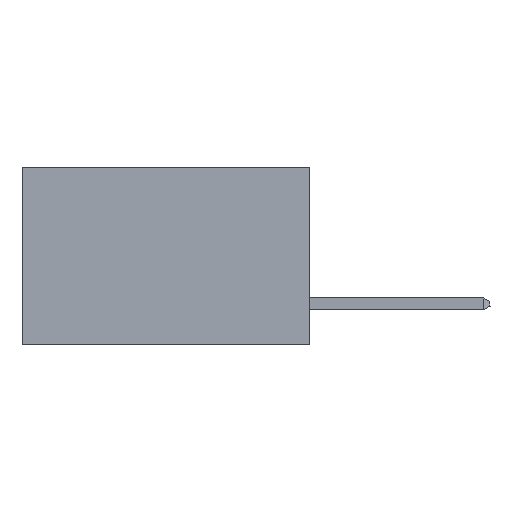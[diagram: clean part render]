
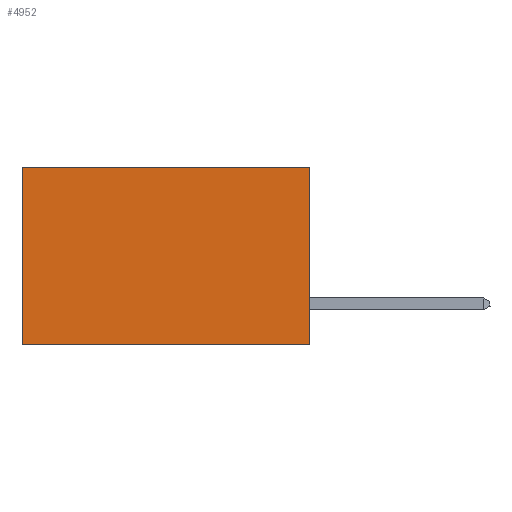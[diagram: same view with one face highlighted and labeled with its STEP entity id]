
A CAD part, left-side view. The second image highlights one B-rep face of the part: STEP entity #4952.
In plain terms, the highlighted planar face has unit normal (-1, 0, 0).
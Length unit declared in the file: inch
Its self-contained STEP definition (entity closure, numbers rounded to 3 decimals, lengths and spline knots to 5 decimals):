
#115 = DIRECTION ( 'NONE',  ( 0., 1., 0. ) ) ;
#611 = ORIENTED_EDGE ( 'NONE', *, *, #8320, .T. ) ;
#1024 = EDGE_CURVE ( 'NONE', #9389, #12700, #13261, .T. ) ;
#1799 = CARTESIAN_POINT ( 'NONE',  ( 0.2875, 0., 0. ) ) ;
#2365 = DIRECTION ( 'NONE',  ( 0., 0., -1. ) ) ;
#3129 = ORIENTED_EDGE ( 'NONE', *, *, #5787, .T. ) ;
#3602 = DIRECTION ( 'NONE',  ( 0., 0., -1. ) ) ;
#3734 = DIRECTION ( 'NONE',  ( 1., 0., 0. ) ) ;
#4619 = PLANE ( 'NONE',  #8424 ) ;
#4673 = ORIENTED_EDGE ( 'NONE', *, *, #1024, .F. ) ;
#4952 = ADVANCED_FACE ( 'NONE', ( #7099 ), #4619, .F. ) ;
#5187 = CARTESIAN_POINT ( 'NONE',  ( 0.2875, 0., 0. ) ) ;
#5602 = VERTEX_POINT ( 'NONE', #5679 ) ;
#5609 = LINE ( 'NONE', #6415, #8518 ) ;
#5679 = CARTESIAN_POINT ( 'NONE',  ( 0.2875, 0.6, 0. ) ) ;
#5787 = EDGE_CURVE ( 'NONE', #9173, #5602, #13251, .T. ) ;
#5986 = VECTOR ( 'NONE', #11693, 39.37008 ) ;
#6407 = DIRECTION ( 'NONE',  ( 0., 1., 0. ) ) ;
#6415 = CARTESIAN_POINT ( 'NONE',  ( 0.2875, 0., 0. ) ) ;
#6842 = VECTOR ( 'NONE', #115, 39.37008 ) ;
#7099 = FACE_OUTER_BOUND ( 'NONE', #7906, .T. ) ;
#7686 = CARTESIAN_POINT ( 'NONE',  ( 0.2875, 0.6, -0.37 ) ) ;
#7906 = EDGE_LOOP ( 'NONE', ( #611, #4673, #9855, #3129 ) ) ;
#8320 = EDGE_CURVE ( 'NONE', #5602, #12700, #11550, .T. ) ;
#8424 = AXIS2_PLACEMENT_3D ( 'NONE', #10837, #3734, #3602 ) ;
#8518 = VECTOR ( 'NONE', #2365, 39.37008 ) ;
#9173 = VERTEX_POINT ( 'NONE', #1799 ) ;
#9389 = VERTEX_POINT ( 'NONE', #12559 ) ;
#9493 = CARTESIAN_POINT ( 'NONE',  ( 0.2875, 0., -0.37 ) ) ;
#9855 = ORIENTED_EDGE ( 'NONE', *, *, #10368, .F. ) ;
#10368 = EDGE_CURVE ( 'NONE', #9173, #9389, #5609, .T. ) ;
#10837 = CARTESIAN_POINT ( 'NONE',  ( 0.2875, 0., 0. ) ) ;
#11550 = LINE ( 'NONE', #13439, #5986 ) ;
#11693 = DIRECTION ( 'NONE',  ( 0., 0., -1. ) ) ;
#12559 = CARTESIAN_POINT ( 'NONE',  ( 0.2875, 0., -0.37 ) ) ;
#12700 = VERTEX_POINT ( 'NONE', #7686 ) ;
#12761 = VECTOR ( 'NONE', #6407, 39.37008 ) ;
#13251 = LINE ( 'NONE', #5187, #6842 ) ;
#13261 = LINE ( 'NONE', #9493, #12761 ) ;
#13439 = CARTESIAN_POINT ( 'NONE',  ( 0.2875, 0.6, 0. ) ) ;
